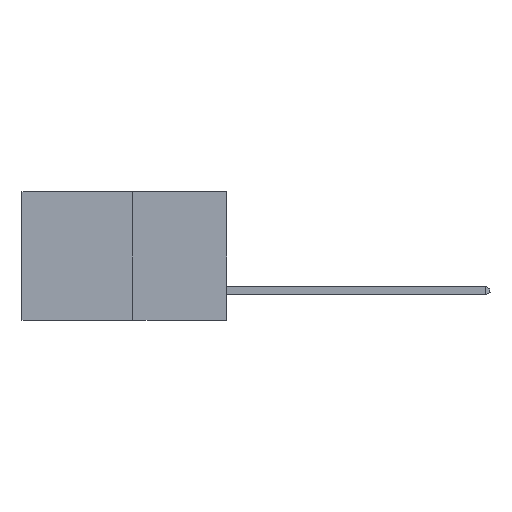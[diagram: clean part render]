
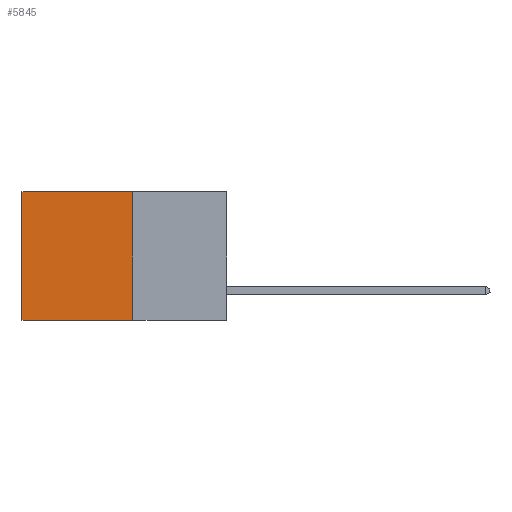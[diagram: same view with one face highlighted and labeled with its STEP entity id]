
A CAD part, left-side view. The second image highlights one B-rep face of the part: STEP entity #5845.
In plain terms, the highlighted planar face has unit normal (-1, 0, 0).
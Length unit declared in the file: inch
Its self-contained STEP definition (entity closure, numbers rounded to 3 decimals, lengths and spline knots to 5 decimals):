
#112 = EDGE_CURVE ( 'NONE', #478, #1700, #6635, .T. ) ;
#194 = CARTESIAN_POINT ( 'NONE',  ( 0.277, 0.59, -0.37 ) ) ;
#478 = VERTEX_POINT ( 'NONE', #9775 ) ;
#968 = CARTESIAN_POINT ( 'NONE',  ( 0.277, 0.27, -0.37 ) ) ;
#977 = VECTOR ( 'NONE', #3327, 39.37008 ) ;
#1213 = DIRECTION ( 'NONE',  ( 0., 0., -1. ) ) ;
#1534 = LINE ( 'NONE', #5408, #8297 ) ;
#1700 = VERTEX_POINT ( 'NONE', #194 ) ;
#1880 = LINE ( 'NONE', #7880, #977 ) ;
#2763 = VECTOR ( 'NONE', #1213, 39.37008 ) ;
#2884 = DIRECTION ( 'NONE',  ( 1., 0., 0. ) ) ;
#2965 = CARTESIAN_POINT ( 'NONE',  ( 0.277, 0.27, 0. ) ) ;
#3187 = VERTEX_POINT ( 'NONE', #2965 ) ;
#3327 = DIRECTION ( 'NONE',  ( 0., 0., -1. ) ) ;
#3826 = DIRECTION ( 'NONE',  ( 0., 1., 0. ) ) ;
#3865 = CARTESIAN_POINT ( 'NONE',  ( 0.277, 0.27, -0.37 ) ) ;
#4097 = EDGE_LOOP ( 'NONE', ( #7725, #10187, #6543, #6160 ) ) ;
#4985 = CARTESIAN_POINT ( 'NONE',  ( 0.277, 0.59, 0. ) ) ;
#5408 = CARTESIAN_POINT ( 'NONE',  ( 0.277, 0.27, 0. ) ) ;
#5555 = PLANE ( 'NONE',  #6380 ) ;
#5780 = CARTESIAN_POINT ( 'NONE',  ( 0.277, 0.59, -0.37 ) ) ;
#5845 = ADVANCED_FACE ( 'NONE', ( #7253 ), #5555, .F. ) ;
#6160 = ORIENTED_EDGE ( 'NONE', *, *, #10229, .T. ) ;
#6317 = DIRECTION ( 'NONE',  ( 0., 1., 0. ) ) ;
#6380 = AXIS2_PLACEMENT_3D ( 'NONE', #968, #2884, #9258 ) ;
#6543 = ORIENTED_EDGE ( 'NONE', *, *, #8590, .F. ) ;
#6635 = LINE ( 'NONE', #3865, #11376 ) ;
#7253 = FACE_OUTER_BOUND ( 'NONE', #4097, .T. ) ;
#7725 = ORIENTED_EDGE ( 'NONE', *, *, #8362, .T. ) ;
#7880 = CARTESIAN_POINT ( 'NONE',  ( 0.277, 0.27, -0.37 ) ) ;
#8297 = VECTOR ( 'NONE', #6317, 39.37008 ) ;
#8362 = EDGE_CURVE ( 'NONE', #8476, #1700, #9997, .T. ) ;
#8476 = VERTEX_POINT ( 'NONE', #4985 ) ;
#8590 = EDGE_CURVE ( 'NONE', #3187, #478, #1880, .T. ) ;
#9258 = DIRECTION ( 'NONE',  ( 0., 0., -1. ) ) ;
#9775 = CARTESIAN_POINT ( 'NONE',  ( 0.277, 0.27, -0.37 ) ) ;
#9997 = LINE ( 'NONE', #5780, #2763 ) ;
#10187 = ORIENTED_EDGE ( 'NONE', *, *, #112, .F. ) ;
#10229 = EDGE_CURVE ( 'NONE', #3187, #8476, #1534, .T. ) ;
#11376 = VECTOR ( 'NONE', #3826, 39.37008 ) ;
